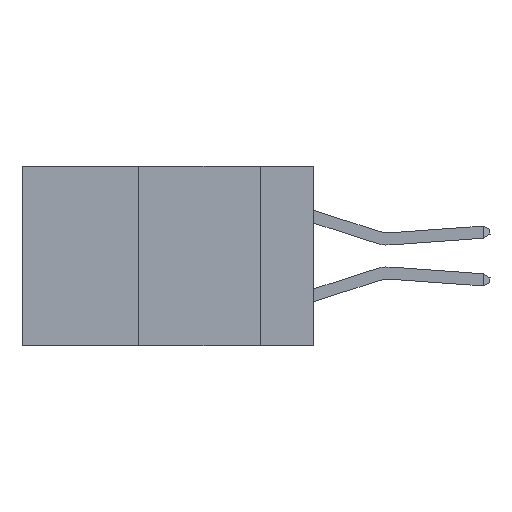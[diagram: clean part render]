
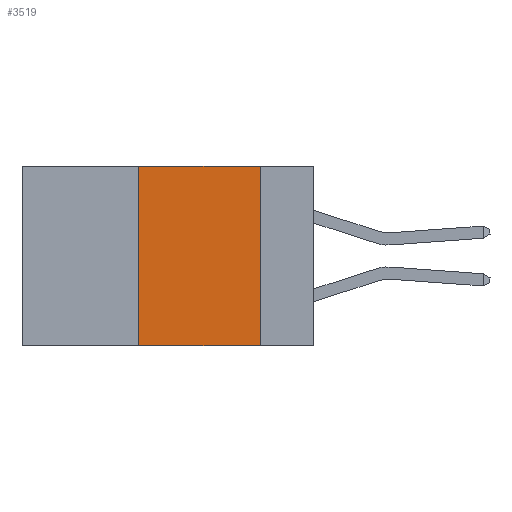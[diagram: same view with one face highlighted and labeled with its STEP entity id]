
A CAD part, left-side view. The second image highlights one B-rep face of the part: STEP entity #3519.
In plain terms, the highlighted planar face has unit normal (-1, 0, 0).
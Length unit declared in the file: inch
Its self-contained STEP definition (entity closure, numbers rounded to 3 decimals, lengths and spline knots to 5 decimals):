
#1762 = VECTOR ( 'NONE', #13640, 39.37008 ) ;
#3222 = CARTESIAN_POINT ( 'NONE',  ( 0., 0.11, 0. ) ) ;
#3297 = LINE ( 'NONE', #3222, #18884 ) ;
#3519 = ADVANCED_FACE ( 'NONE', ( #20340 ), #28352, .F. ) ;
#3597 = CARTESIAN_POINT ( 'NONE',  ( 0., 0.6, -0.37 ) ) ;
#3787 = VERTEX_POINT ( 'NONE', #4075 ) ;
#3830 = CARTESIAN_POINT ( 'NONE',  ( 0., 0.11, -0.37 ) ) ;
#4075 = CARTESIAN_POINT ( 'NONE',  ( 0., 0.11, 0. ) ) ;
#5039 = VERTEX_POINT ( 'NONE', #8085 ) ;
#6615 = ORIENTED_EDGE ( 'NONE', *, *, #7196, .T. ) ;
#7196 = EDGE_CURVE ( 'NONE', #10677, #16242, #10106, .T. ) ;
#7792 = CARTESIAN_POINT ( 'NONE',  ( 0., 0.6, 0. ) ) ;
#8085 = CARTESIAN_POINT ( 'NONE',  ( 0., 0.36, 0. ) ) ;
#8349 = DIRECTION ( 'NONE',  ( 0., 0., -1. ) ) ;
#8698 = VECTOR ( 'NONE', #23270, 39.37008 ) ;
#9921 = DIRECTION ( 'NONE',  ( 0., -1., 0. ) ) ;
#10060 = EDGE_CURVE ( 'NONE', #10677, #5039, #15528, .T. ) ;
#10106 = LINE ( 'NONE', #3597, #1762 ) ;
#10677 = VERTEX_POINT ( 'NONE', #17792 ) ;
#13025 = DIRECTION ( 'NONE',  ( 0., 0., -1. ) ) ;
#13640 = DIRECTION ( 'NONE',  ( 0., -1., 0. ) ) ;
#14330 = EDGE_LOOP ( 'NONE', ( #23978, #21349, #19632, #6615 ) ) ;
#15528 = LINE ( 'NONE', #26196, #8698 ) ;
#15728 = DIRECTION ( 'NONE',  ( 1., 0., 0. ) ) ;
#16242 = VERTEX_POINT ( 'NONE', #3830 ) ;
#17792 = CARTESIAN_POINT ( 'NONE',  ( 0., 0.36, -0.37 ) ) ;
#18884 = VECTOR ( 'NONE', #8349, 39.37008 ) ;
#19632 = ORIENTED_EDGE ( 'NONE', *, *, #10060, .F. ) ;
#20340 = FACE_OUTER_BOUND ( 'NONE', #14330, .T. ) ;
#20567 = VECTOR ( 'NONE', #9921, 39.37008 ) ;
#21349 = ORIENTED_EDGE ( 'NONE', *, *, #27758, .F. ) ;
#21377 = LINE ( 'NONE', #23093, #20567 ) ;
#23093 = CARTESIAN_POINT ( 'NONE',  ( 0., 0.6, 0. ) ) ;
#23270 = DIRECTION ( 'NONE',  ( 0., 0., 1. ) ) ;
#23577 = EDGE_CURVE ( 'NONE', #3787, #16242, #3297, .T. ) ;
#23978 = ORIENTED_EDGE ( 'NONE', *, *, #23577, .F. ) ;
#26196 = CARTESIAN_POINT ( 'NONE',  ( 0., 0.36, 0. ) ) ;
#26456 = AXIS2_PLACEMENT_3D ( 'NONE', #7792, #15728, #13025 ) ;
#27758 = EDGE_CURVE ( 'NONE', #5039, #3787, #21377, .T. ) ;
#28352 = PLANE ( 'NONE',  #26456 ) ;
